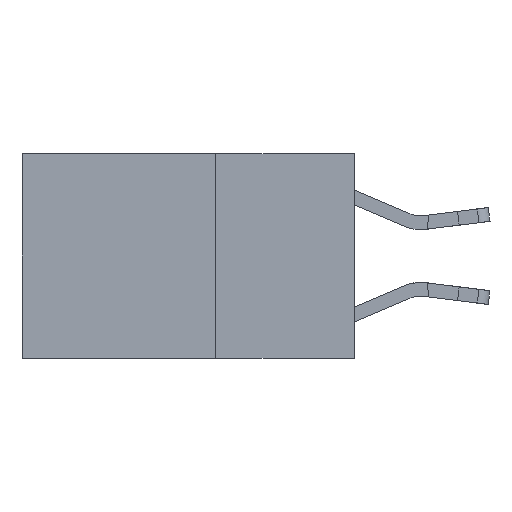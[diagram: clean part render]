
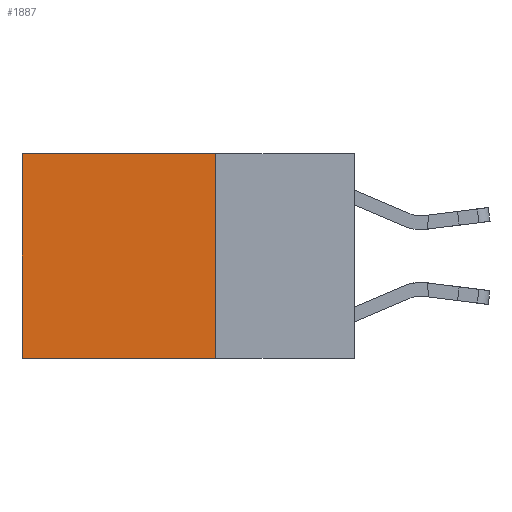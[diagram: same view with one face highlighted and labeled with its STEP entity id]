
A CAD part, left-side view. The second image highlights one B-rep face of the part: STEP entity #1887.
In plain terms, the highlighted planar face has unit normal (-1, 0, 0).
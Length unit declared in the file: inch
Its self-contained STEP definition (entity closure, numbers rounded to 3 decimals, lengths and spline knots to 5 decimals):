
#225 = LINE ( 'NONE', #15999, #12680 ) ;
#933 = ORIENTED_EDGE ( 'NONE', *, *, #5388, .T. ) ;
#1194 = CARTESIAN_POINT ( 'NONE',  ( 0.2625, 0.25, -0.37 ) ) ;
#1707 = LINE ( 'NONE', #16252, #4416 ) ;
#1778 = CARTESIAN_POINT ( 'NONE',  ( 0.2625, 0.25, 0. ) ) ;
#1887 = ADVANCED_FACE ( 'NONE', ( #14601 ), #13309, .F. ) ;
#3628 = CARTESIAN_POINT ( 'NONE',  ( 0.2625, 0.6, 0. ) ) ;
#3990 = EDGE_CURVE ( 'NONE', #13087, #17227, #5625, .T. ) ;
#4246 = DIRECTION ( 'NONE',  ( 0., 0., -1. ) ) ;
#4416 = VECTOR ( 'NONE', #4246, 39.37008 ) ;
#4472 = DIRECTION ( 'NONE',  ( 0., 1., 0. ) ) ;
#4664 = AXIS2_PLACEMENT_3D ( 'NONE', #6630, #15268, #10388 ) ;
#4914 = DIRECTION ( 'NONE',  ( 0., 1., 0. ) ) ;
#5388 = EDGE_CURVE ( 'NONE', #7445, #17227, #1707, .T. ) ;
#5571 = DIRECTION ( 'NONE',  ( 0., 0., -1. ) ) ;
#5625 = LINE ( 'NONE', #8434, #13158 ) ;
#6321 = LINE ( 'NONE', #6589, #16219 ) ;
#6589 = CARTESIAN_POINT ( 'NONE',  ( 0.2625, 0.25, 0. ) ) ;
#6630 = CARTESIAN_POINT ( 'NONE',  ( 0.2625, 0.25, 0. ) ) ;
#6895 = EDGE_LOOP ( 'NONE', ( #933, #10119, #17074, #9656 ) ) ;
#7445 = VERTEX_POINT ( 'NONE', #3628 ) ;
#8434 = CARTESIAN_POINT ( 'NONE',  ( 0.2625, 0.25, -0.37 ) ) ;
#9116 = VERTEX_POINT ( 'NONE', #1778 ) ;
#9656 = ORIENTED_EDGE ( 'NONE', *, *, #10652, .T. ) ;
#10119 = ORIENTED_EDGE ( 'NONE', *, *, #3990, .F. ) ;
#10388 = DIRECTION ( 'NONE',  ( 0., 0., -1. ) ) ;
#10652 = EDGE_CURVE ( 'NONE', #9116, #7445, #6321, .T. ) ;
#12278 = CARTESIAN_POINT ( 'NONE',  ( 0.2625, 0.6, -0.37 ) ) ;
#12680 = VECTOR ( 'NONE', #5571, 39.37008 ) ;
#13064 = EDGE_CURVE ( 'NONE', #9116, #13087, #225, .T. ) ;
#13087 = VERTEX_POINT ( 'NONE', #1194 ) ;
#13158 = VECTOR ( 'NONE', #4472, 39.37008 ) ;
#13309 = PLANE ( 'NONE',  #4664 ) ;
#14601 = FACE_OUTER_BOUND ( 'NONE', #6895, .T. ) ;
#15268 = DIRECTION ( 'NONE',  ( 1., 0., 0. ) ) ;
#15999 = CARTESIAN_POINT ( 'NONE',  ( 0.2625, 0.25, 0. ) ) ;
#16219 = VECTOR ( 'NONE', #4914, 39.37008 ) ;
#16252 = CARTESIAN_POINT ( 'NONE',  ( 0.2625, 0.6, 0. ) ) ;
#17074 = ORIENTED_EDGE ( 'NONE', *, *, #13064, .F. ) ;
#17227 = VERTEX_POINT ( 'NONE', #12278 ) ;
